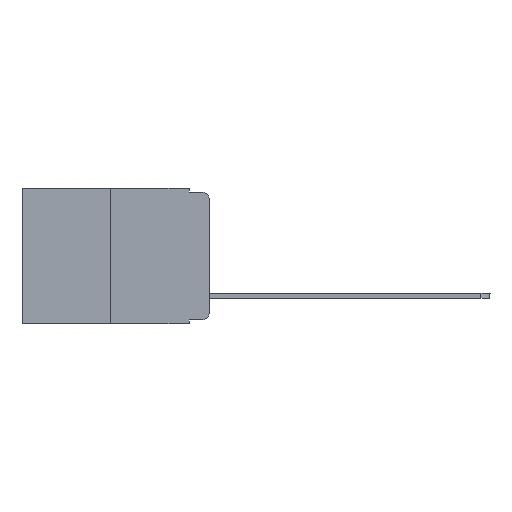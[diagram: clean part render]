
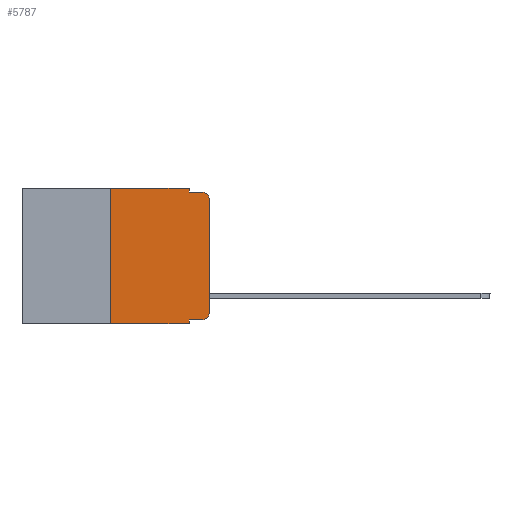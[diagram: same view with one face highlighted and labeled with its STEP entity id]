
A CAD part, left-side view. The second image highlights one B-rep face of the part: STEP entity #5787.
In plain terms, the highlighted planar face has unit normal (-1, 0, 0).
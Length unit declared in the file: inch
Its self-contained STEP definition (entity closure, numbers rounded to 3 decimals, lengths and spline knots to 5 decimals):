
#413 = FACE_OUTER_BOUND ( 'NONE', #9507, .T. ) ;
#490 = ORIENTED_EDGE ( 'NONE', *, *, #8023, .F. ) ;
#677 = VERTEX_POINT ( 'NONE', #4938 ) ;
#846 = VERTEX_POINT ( 'NONE', #10396 ) ;
#983 = CARTESIAN_POINT ( 'NONE',  ( 0., 0., 0. ) ) ;
#1136 = VERTEX_POINT ( 'NONE', #6094 ) ;
#1356 = DIRECTION ( 'NONE',  ( 0., 0., -1. ) ) ;
#1489 = LINE ( 'NONE', #5316, #8169 ) ;
#1620 = DIRECTION ( 'NONE',  ( 0., 0., 1. ) ) ;
#1754 = VECTOR ( 'NONE', #10451, 39.37008 ) ;
#2085 = EDGE_CURVE ( 'NONE', #846, #12159, #2948, .T. ) ;
#2348 = EDGE_CURVE ( 'NONE', #8841, #677, #8361, .T. ) ;
#2927 = CARTESIAN_POINT ( 'NONE',  ( 0., 0.02, -0.03 ) ) ;
#2948 = CIRCLE ( 'NONE', #3909, 0.02 ) ;
#3119 = DIRECTION ( 'NONE',  ( -1., 0., 0. ) ) ;
#3154 = CARTESIAN_POINT ( 'NONE',  ( 0., 0.051, -0.333 ) ) ;
#3255 = ORIENTED_EDGE ( 'NONE', *, *, #7700, .T. ) ;
#3293 = EDGE_CURVE ( 'NONE', #9182, #9529, #9614, .T. ) ;
#3570 = VECTOR ( 'NONE', #1620, 39.37008 ) ;
#3640 = VECTOR ( 'NONE', #7115, 39.37008 ) ;
#3698 = LINE ( 'NONE', #5452, #8340 ) ;
#3727 = ORIENTED_EDGE ( 'NONE', *, *, #5772, .F. ) ;
#3807 = DIRECTION ( 'NONE',  ( -1., 0., 0. ) ) ;
#3909 = AXIS2_PLACEMENT_3D ( 'NONE', #9091, #3119, #10099 ) ;
#4025 = LINE ( 'NONE', #983, #8513 ) ;
#4449 = EDGE_CURVE ( 'NONE', #12159, #9182, #4025, .T. ) ;
#4503 = CARTESIAN_POINT ( 'NONE',  ( 0., 0.051, 0. ) ) ;
#4938 = CARTESIAN_POINT ( 'NONE',  ( 0., 0.25, 0. ) ) ;
#4987 = CARTESIAN_POINT ( 'NONE',  ( 0., 0.051, -0.343 ) ) ;
#5234 = EDGE_CURVE ( 'NONE', #1136, #9529, #3698, .T. ) ;
#5316 = CARTESIAN_POINT ( 'NONE',  ( 0., 0.473, 0. ) ) ;
#5452 = CARTESIAN_POINT ( 'NONE',  ( 0., 0.051, -0.01 ) ) ;
#5608 = ORIENTED_EDGE ( 'NONE', *, *, #4449, .T. ) ;
#5670 = DIRECTION ( 'NONE',  ( 0., -1., 0. ) ) ;
#5772 = EDGE_CURVE ( 'NONE', #677, #7397, #1489, .T. ) ;
#5787 = ADVANCED_FACE ( 'NONE', ( #413 ), #7211, .F. ) ;
#5864 = CARTESIAN_POINT ( 'NONE',  ( 0., 0.25, -0.343 ) ) ;
#5912 = AXIS2_PLACEMENT_3D ( 'NONE', #7342, #7382, #1356 ) ;
#5948 = LINE ( 'NONE', #10620, #8413 ) ;
#6094 = CARTESIAN_POINT ( 'NONE',  ( 0., 0.051, -0.01 ) ) ;
#6165 = CARTESIAN_POINT ( 'NONE',  ( 0., 0., -0.313 ) ) ;
#6206 = DIRECTION ( 'NONE',  ( 0., -1., 0. ) ) ;
#6897 = LINE ( 'NONE', #3154, #3640 ) ;
#6925 = VERTEX_POINT ( 'NONE', #10832 ) ;
#7115 = DIRECTION ( 'NONE',  ( 0., -1., 0. ) ) ;
#7211 = PLANE ( 'NONE',  #5912 ) ;
#7342 = CARTESIAN_POINT ( 'NONE',  ( 0., 0.473, 0. ) ) ;
#7382 = DIRECTION ( 'NONE',  ( 1., 0., 0. ) ) ;
#7397 = VERTEX_POINT ( 'NONE', #11455 ) ;
#7539 = ORIENTED_EDGE ( 'NONE', *, *, #3293, .T. ) ;
#7700 = EDGE_CURVE ( 'NONE', #6925, #846, #6897, .T. ) ;
#7820 = CARTESIAN_POINT ( 'NONE',  ( 0., 0.02, -0.01 ) ) ;
#7930 = LINE ( 'NONE', #10337, #10286 ) ;
#8023 = EDGE_CURVE ( 'NONE', #6925, #10077, #10343, .T. ) ;
#8131 = ORIENTED_EDGE ( 'NONE', *, *, #5234, .F. ) ;
#8169 = VECTOR ( 'NONE', #6206, 39.37008 ) ;
#8314 = ORIENTED_EDGE ( 'NONE', *, *, #2348, .F. ) ;
#8340 = VECTOR ( 'NONE', #5670, 39.37008 ) ;
#8361 = LINE ( 'NONE', #11481, #3570 ) ;
#8370 = AXIS2_PLACEMENT_3D ( 'NONE', #2927, #3807, #8833 ) ;
#8413 = VECTOR ( 'NONE', #9546, 39.37008 ) ;
#8513 = VECTOR ( 'NONE', #9823, 39.37008 ) ;
#8833 = DIRECTION ( 'NONE',  ( 0., 0., -1. ) ) ;
#8841 = VERTEX_POINT ( 'NONE', #5864 ) ;
#9091 = CARTESIAN_POINT ( 'NONE',  ( 0., 0.02, -0.313 ) ) ;
#9182 = VERTEX_POINT ( 'NONE', #9439 ) ;
#9251 = ORIENTED_EDGE ( 'NONE', *, *, #2085, .T. ) ;
#9439 = CARTESIAN_POINT ( 'NONE',  ( 0., 0., -0.03 ) ) ;
#9489 = DIRECTION ( 'NONE',  ( 0., -1., 0. ) ) ;
#9507 = EDGE_LOOP ( 'NONE', ( #5608, #7539, #8131, #11136, #3727, #8314, #12069, #490, #3255, #9251 ) ) ;
#9529 = VERTEX_POINT ( 'NONE', #7820 ) ;
#9546 = DIRECTION ( 'NONE',  ( 0., 0., -1. ) ) ;
#9614 = CIRCLE ( 'NONE', #8370, 0.02 ) ;
#9621 = EDGE_CURVE ( 'NONE', #8841, #10077, #7930, .T. ) ;
#9823 = DIRECTION ( 'NONE',  ( 0., 0., 1. ) ) ;
#10077 = VERTEX_POINT ( 'NONE', #4987 ) ;
#10099 = DIRECTION ( 'NONE',  ( 0., 0., -1. ) ) ;
#10286 = VECTOR ( 'NONE', #9489, 39.37008 ) ;
#10337 = CARTESIAN_POINT ( 'NONE',  ( 0., 0.473, -0.343 ) ) ;
#10343 = LINE ( 'NONE', #4503, #1754 ) ;
#10396 = CARTESIAN_POINT ( 'NONE',  ( 0., 0.02, -0.333 ) ) ;
#10451 = DIRECTION ( 'NONE',  ( 0., 0., -1. ) ) ;
#10620 = CARTESIAN_POINT ( 'NONE',  ( 0., 0.051, 0. ) ) ;
#10832 = CARTESIAN_POINT ( 'NONE',  ( 0., 0.051, -0.333 ) ) ;
#10991 = EDGE_CURVE ( 'NONE', #7397, #1136, #5948, .T. ) ;
#11136 = ORIENTED_EDGE ( 'NONE', *, *, #10991, .F. ) ;
#11455 = CARTESIAN_POINT ( 'NONE',  ( 0., 0.051, 0. ) ) ;
#11481 = CARTESIAN_POINT ( 'NONE',  ( 0., 0.25, 0. ) ) ;
#12069 = ORIENTED_EDGE ( 'NONE', *, *, #9621, .T. ) ;
#12159 = VERTEX_POINT ( 'NONE', #6165 ) ;
